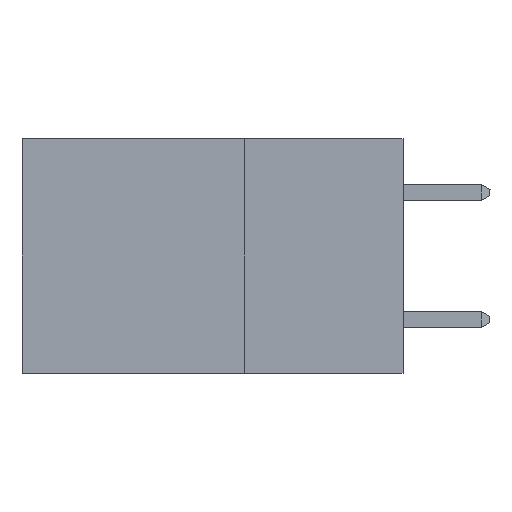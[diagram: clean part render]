
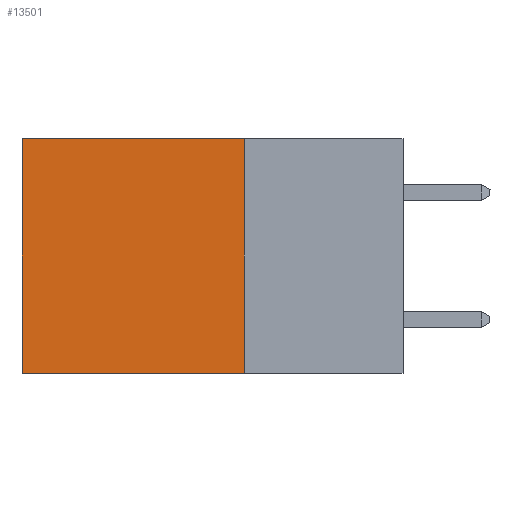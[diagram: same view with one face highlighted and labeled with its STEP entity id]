
A CAD part, left-side view. The second image highlights one B-rep face of the part: STEP entity #13501.
In plain terms, the highlighted planar face has unit normal (-1, 0, 0).
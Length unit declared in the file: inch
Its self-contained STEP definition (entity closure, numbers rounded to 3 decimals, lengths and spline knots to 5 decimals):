
#305 = VECTOR ( 'NONE', #29309, 39.37008 ) ;
#549 = DIRECTION ( 'NONE',  ( 0., 0., -1. ) ) ;
#1274 = EDGE_CURVE ( 'NONE', #6251, #1514, #42713, .T. ) ;
#1514 = VERTEX_POINT ( 'NONE', #13278 ) ;
#2001 = CARTESIAN_POINT ( 'NONE',  ( 0.2875, 0.25, -0.37 ) ) ;
#2304 = VECTOR ( 'NONE', #39716, 39.37008 ) ;
#6251 = VERTEX_POINT ( 'NONE', #29150 ) ;
#6314 = VERTEX_POINT ( 'NONE', #42785 ) ;
#9221 = LINE ( 'NONE', #25970, #305 ) ;
#9232 = AXIS2_PLACEMENT_3D ( 'NONE', #17293, #20709, #549 ) ;
#10206 = LINE ( 'NONE', #15425, #27005 ) ;
#13027 = CARTESIAN_POINT ( 'NONE',  ( 0.2875, 0.25, 0. ) ) ;
#13278 = CARTESIAN_POINT ( 'NONE',  ( 0.2875, 0.6, -0.37 ) ) ;
#13501 = ADVANCED_FACE ( 'NONE', ( #36425 ), #37241, .F. ) ;
#13828 = EDGE_LOOP ( 'NONE', ( #34647, #28620, #34484, #27429 ) ) ;
#15425 = CARTESIAN_POINT ( 'NONE',  ( 0.2875, 0.6, 0. ) ) ;
#16136 = VECTOR ( 'NONE', #38674, 39.37008 ) ;
#16634 = EDGE_CURVE ( 'NONE', #6314, #36041, #9221, .T. ) ;
#17293 = CARTESIAN_POINT ( 'NONE',  ( 0.2875, 0.25, 0. ) ) ;
#20318 = EDGE_CURVE ( 'NONE', #36041, #1514, #10206, .T. ) ;
#20709 = DIRECTION ( 'NONE',  ( 1., 0., 0. ) ) ;
#21244 = LINE ( 'NONE', #13027, #2304 ) ;
#25970 = CARTESIAN_POINT ( 'NONE',  ( 0.2875, 0.25, 0. ) ) ;
#27005 = VECTOR ( 'NONE', #35395, 39.37008 ) ;
#27429 = ORIENTED_EDGE ( 'NONE', *, *, #16634, .T. ) ;
#28032 = CARTESIAN_POINT ( 'NONE',  ( 0.2875, 0.6, 0. ) ) ;
#28620 = ORIENTED_EDGE ( 'NONE', *, *, #1274, .F. ) ;
#29150 = CARTESIAN_POINT ( 'NONE',  ( 0.2875, 0.25, -0.37 ) ) ;
#29309 = DIRECTION ( 'NONE',  ( 0., 1., 0. ) ) ;
#34484 = ORIENTED_EDGE ( 'NONE', *, *, #38410, .F. ) ;
#34647 = ORIENTED_EDGE ( 'NONE', *, *, #20318, .T. ) ;
#35395 = DIRECTION ( 'NONE',  ( 0., 0., -1. ) ) ;
#36041 = VERTEX_POINT ( 'NONE', #28032 ) ;
#36425 = FACE_OUTER_BOUND ( 'NONE', #13828, .T. ) ;
#37241 = PLANE ( 'NONE',  #9232 ) ;
#38410 = EDGE_CURVE ( 'NONE', #6314, #6251, #21244, .T. ) ;
#38674 = DIRECTION ( 'NONE',  ( 0., 1., 0. ) ) ;
#39716 = DIRECTION ( 'NONE',  ( 0., 0., -1. ) ) ;
#42713 = LINE ( 'NONE', #2001, #16136 ) ;
#42785 = CARTESIAN_POINT ( 'NONE',  ( 0.2875, 0.25, 0. ) ) ;
